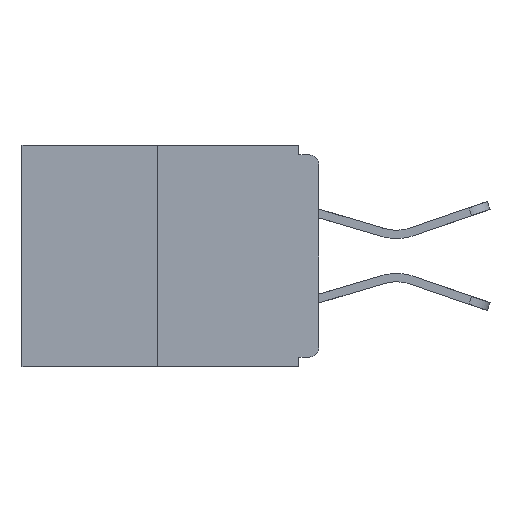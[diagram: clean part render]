
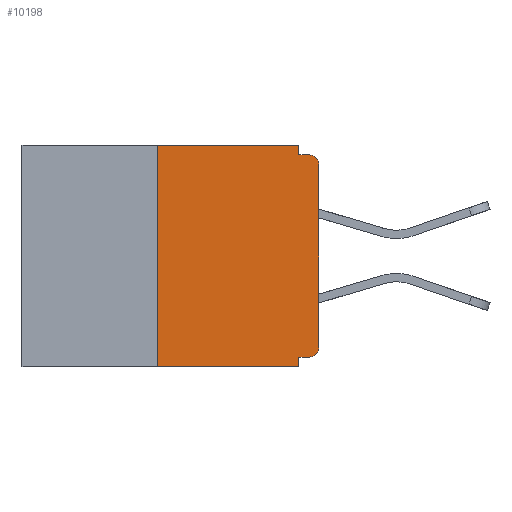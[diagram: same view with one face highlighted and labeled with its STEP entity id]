
A CAD part, left-side view. The second image highlights one B-rep face of the part: STEP entity #10198.
In plain terms, the highlighted planar face has unit normal (-1, 0, 0).
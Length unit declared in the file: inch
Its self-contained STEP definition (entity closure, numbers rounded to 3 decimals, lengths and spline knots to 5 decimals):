
#639 = LINE ( 'NONE', #9751, #20464 ) ;
#806 = LINE ( 'NONE', #18347, #13475 ) ;
#1145 = EDGE_CURVE ( 'NONE', #23285, #27194, #21402, .T. ) ;
#1209 = CARTESIAN_POINT ( 'NONE',  ( 0., 0.25, 0. ) ) ;
#1281 = LINE ( 'NONE', #13689, #2838 ) ;
#1858 = ORIENTED_EDGE ( 'NONE', *, *, #31153, .F. ) ;
#2161 = VERTEX_POINT ( 'NONE', #26321 ) ;
#2208 = VECTOR ( 'NONE', #19322, 39.37008 ) ;
#2444 = EDGE_LOOP ( 'NONE', ( #23940, #9740, #2449, #31008, #1858, #25133, #22364, #23691, #9396, #32028 ) ) ;
#2449 = ORIENTED_EDGE ( 'NONE', *, *, #32146, .T. ) ;
#2838 = VECTOR ( 'NONE', #6169, 39.37008 ) ;
#4019 = DIRECTION ( 'NONE',  ( 0., -1., 0. ) ) ;
#4542 = VERTEX_POINT ( 'NONE', #22145 ) ;
#5081 = FACE_OUTER_BOUND ( 'NONE', #2444, .T. ) ;
#6151 = CARTESIAN_POINT ( 'NONE',  ( 0., 0., 0. ) ) ;
#6169 = DIRECTION ( 'NONE',  ( 0., 0., 1. ) ) ;
#6257 = DIRECTION ( 'NONE',  ( 0., 0., 1. ) ) ;
#6313 = VECTOR ( 'NONE', #6257, 39.37008 ) ;
#7251 = CIRCLE ( 'NONE', #14016, 0.015 ) ;
#7462 = CARTESIAN_POINT ( 'NONE',  ( 0., 0.031, -0.343 ) ) ;
#7646 = DIRECTION ( 'NONE',  ( -1., 0., 0. ) ) ;
#8981 = DIRECTION ( 'NONE',  ( 0., -1., 0. ) ) ;
#9337 = EDGE_CURVE ( 'NONE', #11178, #23901, #806, .T. ) ;
#9396 = ORIENTED_EDGE ( 'NONE', *, *, #18864, .F. ) ;
#9740 = ORIENTED_EDGE ( 'NONE', *, *, #27958, .F. ) ;
#9751 = CARTESIAN_POINT ( 'NONE',  ( 0., 0., -0.328 ) ) ;
#10176 = CARTESIAN_POINT ( 'NONE',  ( 0., 0., -0.313 ) ) ;
#10198 = ADVANCED_FACE ( 'NONE', ( #5081 ), #22109, .F. ) ;
#10544 = CARTESIAN_POINT ( 'NONE',  ( 0., 0.031, -0.343 ) ) ;
#11178 = VERTEX_POINT ( 'NONE', #1209 ) ;
#12726 = DIRECTION ( 'NONE',  ( 0., 0., -1. ) ) ;
#13475 = VECTOR ( 'NONE', #23272, 39.37008 ) ;
#13612 = CIRCLE ( 'NONE', #31963, 0.015 ) ;
#13689 = CARTESIAN_POINT ( 'NONE',  ( 0., 0.25, 0. ) ) ;
#13749 = VERTEX_POINT ( 'NONE', #18450 ) ;
#14016 = AXIS2_PLACEMENT_3D ( 'NONE', #19293, #31611, #24362 ) ;
#14106 = CARTESIAN_POINT ( 'NONE',  ( 0., 0.46, -0.343 ) ) ;
#15473 = CARTESIAN_POINT ( 'NONE',  ( 0., 0.031, 0. ) ) ;
#15961 = LINE ( 'NONE', #14106, #20006 ) ;
#16624 = CARTESIAN_POINT ( 'NONE',  ( 0., 0.031, 0. ) ) ;
#17517 = EDGE_CURVE ( 'NONE', #23901, #4542, #22432, .T. ) ;
#18311 = VECTOR ( 'NONE', #8981, 39.37008 ) ;
#18347 = CARTESIAN_POINT ( 'NONE',  ( 0., 0.46, 0. ) ) ;
#18450 = CARTESIAN_POINT ( 'NONE',  ( 0., 0.015, -0.328 ) ) ;
#18478 = VERTEX_POINT ( 'NONE', #29431 ) ;
#18864 = EDGE_CURVE ( 'NONE', #4542, #28554, #25913, .T. ) ;
#19293 = CARTESIAN_POINT ( 'NONE',  ( 0., 0.015, -0.03 ) ) ;
#19322 = DIRECTION ( 'NONE',  ( 0., 0., -1. ) ) ;
#20006 = VECTOR ( 'NONE', #4019, 39.37008 ) ;
#20464 = VECTOR ( 'NONE', #27544, 39.37008 ) ;
#20733 = DIRECTION ( 'NONE',  ( 0., 0., -1. ) ) ;
#21097 = VERTEX_POINT ( 'NONE', #7462 ) ;
#21154 = CARTESIAN_POINT ( 'NONE',  ( 0., 0., -0.015 ) ) ;
#21402 = LINE ( 'NONE', #6151, #6313 ) ;
#21678 = EDGE_CURVE ( 'NONE', #2161, #21097, #25760, .T. ) ;
#22109 = PLANE ( 'NONE',  #23970 ) ;
#22145 = CARTESIAN_POINT ( 'NONE',  ( 0., 0.031, -0.015 ) ) ;
#22364 = ORIENTED_EDGE ( 'NONE', *, *, #1145, .T. ) ;
#22432 = LINE ( 'NONE', #16624, #2208 ) ;
#22973 = CARTESIAN_POINT ( 'NONE',  ( 0., 0.015, -0.313 ) ) ;
#23272 = DIRECTION ( 'NONE',  ( 0., -1., 0. ) ) ;
#23285 = VERTEX_POINT ( 'NONE', #10176 ) ;
#23691 = ORIENTED_EDGE ( 'NONE', *, *, #27712, .T. ) ;
#23901 = VERTEX_POINT ( 'NONE', #15473 ) ;
#23940 = ORIENTED_EDGE ( 'NONE', *, *, #9337, .F. ) ;
#23970 = AXIS2_PLACEMENT_3D ( 'NONE', #29753, #30188, #25543 ) ;
#24362 = DIRECTION ( 'NONE',  ( 0., 0., -1. ) ) ;
#24865 = CARTESIAN_POINT ( 'NONE',  ( 0., 0.015, -0.015 ) ) ;
#25133 = ORIENTED_EDGE ( 'NONE', *, *, #32295, .T. ) ;
#25543 = DIRECTION ( 'NONE',  ( 0., 0., -1. ) ) ;
#25760 = LINE ( 'NONE', #10544, #31674 ) ;
#25913 = LINE ( 'NONE', #21154, #18311 ) ;
#26321 = CARTESIAN_POINT ( 'NONE',  ( 0., 0.031, -0.328 ) ) ;
#27194 = VERTEX_POINT ( 'NONE', #28853 ) ;
#27544 = DIRECTION ( 'NONE',  ( 0., 1., 0. ) ) ;
#27712 = EDGE_CURVE ( 'NONE', #27194, #28554, #7251, .T. ) ;
#27958 = EDGE_CURVE ( 'NONE', #18478, #11178, #1281, .T. ) ;
#28554 = VERTEX_POINT ( 'NONE', #24865 ) ;
#28853 = CARTESIAN_POINT ( 'NONE',  ( 0., 0., -0.03 ) ) ;
#29431 = CARTESIAN_POINT ( 'NONE',  ( 0., 0.25, -0.343 ) ) ;
#29753 = CARTESIAN_POINT ( 'NONE',  ( 0., 0.46, 0. ) ) ;
#30188 = DIRECTION ( 'NONE',  ( 1., 0., 0. ) ) ;
#31008 = ORIENTED_EDGE ( 'NONE', *, *, #21678, .F. ) ;
#31153 = EDGE_CURVE ( 'NONE', #13749, #2161, #639, .T. ) ;
#31611 = DIRECTION ( 'NONE',  ( -1., 0., 0. ) ) ;
#31674 = VECTOR ( 'NONE', #20733, 39.37008 ) ;
#31963 = AXIS2_PLACEMENT_3D ( 'NONE', #22973, #7646, #12726 ) ;
#32028 = ORIENTED_EDGE ( 'NONE', *, *, #17517, .F. ) ;
#32146 = EDGE_CURVE ( 'NONE', #18478, #21097, #15961, .T. ) ;
#32295 = EDGE_CURVE ( 'NONE', #13749, #23285, #13612, .T. ) ;
